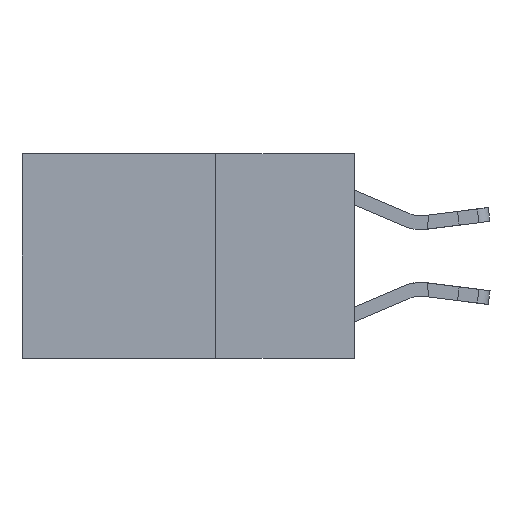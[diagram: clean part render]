
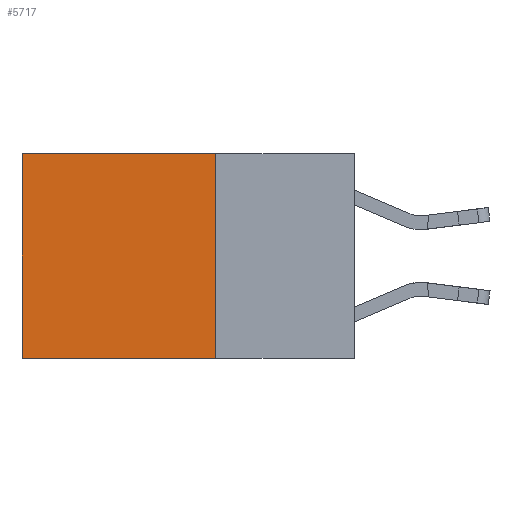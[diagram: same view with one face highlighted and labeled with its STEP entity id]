
A CAD part, left-side view. The second image highlights one B-rep face of the part: STEP entity #5717.
In plain terms, the highlighted planar face has unit normal (-1, 0, 0).
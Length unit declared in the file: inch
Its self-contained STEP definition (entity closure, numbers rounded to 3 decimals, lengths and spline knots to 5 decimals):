
#449 = LINE ( 'NONE', #12966, #11680 ) ;
#711 = AXIS2_PLACEMENT_3D ( 'NONE', #10157, #1719, #16302 ) ;
#814 = EDGE_CURVE ( 'NONE', #21552, #5454, #19480, .T. ) ;
#1702 = CARTESIAN_POINT ( 'NONE',  ( 0.2625, 0.6, 0. ) ) ;
#1719 = DIRECTION ( 'NONE',  ( 1., 0., 0. ) ) ;
#4294 = CARTESIAN_POINT ( 'NONE',  ( 0.2625, 0.25, 0. ) ) ;
#5454 = VERTEX_POINT ( 'NONE', #7258 ) ;
#5717 = ADVANCED_FACE ( 'NONE', ( #5877 ), #14258, .F. ) ;
#5857 = EDGE_CURVE ( 'NONE', #21552, #14650, #23797, .T. ) ;
#5877 = FACE_OUTER_BOUND ( 'NONE', #26641, .T. ) ;
#7031 = ORIENTED_EDGE ( 'NONE', *, *, #814, .T. ) ;
#7258 = CARTESIAN_POINT ( 'NONE',  ( 0.2625, 0.6, 0. ) ) ;
#7508 = VECTOR ( 'NONE', #20816, 39.37008 ) ;
#8111 = DIRECTION ( 'NONE',  ( 0., 1., 0. ) ) ;
#10157 = CARTESIAN_POINT ( 'NONE',  ( 0.2625, 0.25, 0. ) ) ;
#11029 = CARTESIAN_POINT ( 'NONE',  ( 0.2625, 0.25, -0.37 ) ) ;
#11060 = VERTEX_POINT ( 'NONE', #20386 ) ;
#11680 = VECTOR ( 'NONE', #21043, 39.37008 ) ;
#12396 = CARTESIAN_POINT ( 'NONE',  ( 0.2625, 0.25, 0. ) ) ;
#12966 = CARTESIAN_POINT ( 'NONE',  ( 0.2625, 0.25, -0.37 ) ) ;
#14258 = PLANE ( 'NONE',  #711 ) ;
#14650 = VERTEX_POINT ( 'NONE', #11029 ) ;
#16302 = DIRECTION ( 'NONE',  ( 0., 0., -1. ) ) ;
#16418 = EDGE_CURVE ( 'NONE', #5454, #11060, #25845, .T. ) ;
#16517 = ORIENTED_EDGE ( 'NONE', *, *, #5857, .F. ) ;
#16975 = CARTESIAN_POINT ( 'NONE',  ( 0.2625, 0.25, 0. ) ) ;
#18249 = ORIENTED_EDGE ( 'NONE', *, *, #16418, .T. ) ;
#19480 = LINE ( 'NONE', #16975, #24239 ) ;
#20386 = CARTESIAN_POINT ( 'NONE',  ( 0.2625, 0.6, -0.37 ) ) ;
#20478 = VECTOR ( 'NONE', #22415, 39.37008 ) ;
#20816 = DIRECTION ( 'NONE',  ( 0., 0., -1. ) ) ;
#21043 = DIRECTION ( 'NONE',  ( 0., 1., 0. ) ) ;
#21552 = VERTEX_POINT ( 'NONE', #12396 ) ;
#22071 = ORIENTED_EDGE ( 'NONE', *, *, #26045, .F. ) ;
#22415 = DIRECTION ( 'NONE',  ( 0., 0., -1. ) ) ;
#23797 = LINE ( 'NONE', #4294, #7508 ) ;
#24239 = VECTOR ( 'NONE', #8111, 39.37008 ) ;
#25845 = LINE ( 'NONE', #1702, #20478 ) ;
#26045 = EDGE_CURVE ( 'NONE', #14650, #11060, #449, .T. ) ;
#26641 = EDGE_LOOP ( 'NONE', ( #18249, #22071, #16517, #7031 ) ) ;
